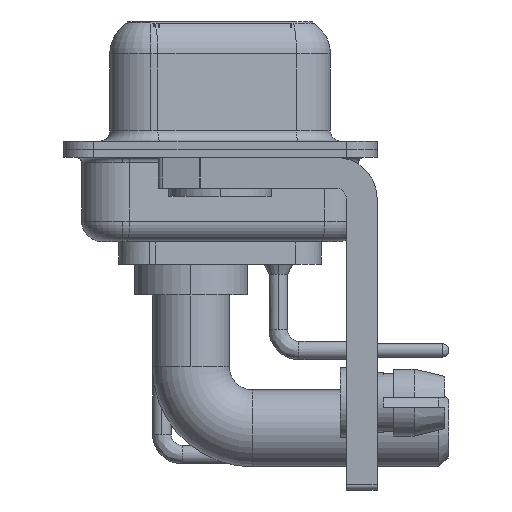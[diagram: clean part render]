
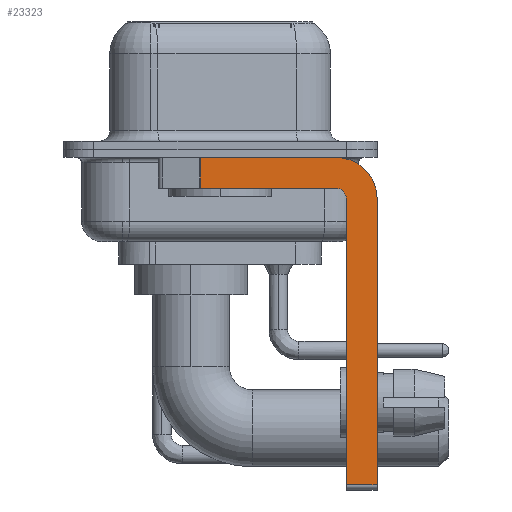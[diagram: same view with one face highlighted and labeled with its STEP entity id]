
A CAD part, left-side view. The second image highlights one B-rep face of the part: STEP entity #23323.
In plain terms, the highlighted planar face has unit normal (-1, 0, 0).
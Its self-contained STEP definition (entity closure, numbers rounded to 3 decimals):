
#7 = LINE ( 'NONE', #16936, #26356 ) ;
#57 = LINE ( 'NONE', #28210, #3231 ) ;
#2900 = LINE ( 'NONE', #16888, #9884 ) ;
#2935 = EDGE_CURVE ( 'NONE', #34196, #8139, #23715, .T. ) ;
#3175 = DIRECTION ( 'NONE',  ( 0., 0., -1. ) ) ;
#3231 = VECTOR ( 'NONE', #3175, 1000. ) ;
#3431 = LINE ( 'NONE', #31217, #35731 ) ;
#4586 = VERTEX_POINT ( 'NONE', #32590 ) ;
#6337 = DIRECTION ( 'NONE',  ( 1., 0., 0. ) ) ;
#8139 = VERTEX_POINT ( 'NONE', #9916 ) ;
#8409 = EDGE_CURVE ( 'NONE', #8139, #26697, #35585, .T. ) ;
#8509 = ORIENTED_EDGE ( 'NONE', *, *, #2935, .F. ) ;
#8805 = ORIENTED_EDGE ( 'NONE', *, *, #31006, .T. ) ;
#9224 = ORIENTED_EDGE ( 'NONE', *, *, #30362, .F. ) ;
#9511 = LINE ( 'NONE', #31940, #32797 ) ;
#9884 = VECTOR ( 'NONE', #13933, 1000. ) ;
#9916 = CARTESIAN_POINT ( 'NONE',  ( -2.9, -5.65, -1.9 ) ) ;
#11908 = EDGE_LOOP ( 'NONE', ( #35743, #8805, #30352, #8509, #9224, #20999, #24292, #25877 ) ) ;
#12571 = DIRECTION ( 'NONE',  ( 0., 0., 1. ) ) ;
#12750 = CARTESIAN_POINT ( 'NONE',  ( -2.9, -5.65, -2.4 ) ) ;
#13039 = CARTESIAN_POINT ( 'NONE',  ( -2.9, -6.15, -2.4 ) ) ;
#13574 = CARTESIAN_POINT ( 'NONE',  ( -2.9, 0.978, -0.4 ) ) ;
#13933 = DIRECTION ( 'NONE',  ( 0., -1., 0. ) ) ;
#14317 = VERTEX_POINT ( 'NONE', #29130 ) ;
#14718 = DIRECTION ( 'NONE',  ( 1., 0., 0. ) ) ;
#15345 = DIRECTION ( 'NONE',  ( -1., 0., 0. ) ) ;
#16706 = DIRECTION ( 'NONE',  ( 0., 0., -1. ) ) ;
#16888 = CARTESIAN_POINT ( 'NONE',  ( -2.9, 3., -0.4 ) ) ;
#16936 = CARTESIAN_POINT ( 'NONE',  ( -2.9, -5.65, -16.35 ) ) ;
#17469 = DIRECTION ( 'NONE',  ( 0., -1., 0. ) ) ;
#18126 = PLANE ( 'NONE',  #21367 ) ;
#18497 = CARTESIAN_POINT ( 'NONE',  ( -2.9, -5.65, -1.9 ) ) ;
#20999 = ORIENTED_EDGE ( 'NONE', *, *, #29851, .T. ) ;
#21367 = AXIS2_PLACEMENT_3D ( 'NONE', #34472, #6337, #31909 ) ;
#21438 = DIRECTION ( 'NONE',  ( 0., 1., 0. ) ) ;
#23323 = ADVANCED_FACE ( 'NONE', ( #31720 ), #18126, .F. ) ;
#23715 = CIRCLE ( 'NONE', #26673, 0.5 ) ;
#24292 = ORIENTED_EDGE ( 'NONE', *, *, #28803, .F. ) ;
#25566 = EDGE_CURVE ( 'NONE', #4586, #31012, #35509, .T. ) ;
#25877 = ORIENTED_EDGE ( 'NONE', *, *, #25566, .F. ) ;
#26356 = VECTOR ( 'NONE', #17469, 1000. ) ;
#26673 = AXIS2_PLACEMENT_3D ( 'NONE', #12750, #15345, #12571 ) ;
#26697 = VERTEX_POINT ( 'NONE', #32928 ) ;
#28210 = CARTESIAN_POINT ( 'NONE',  ( -2.9, 0.978, -1.9 ) ) ;
#28700 = DIRECTION ( 'NONE',  ( 0., 0., -1. ) ) ;
#28803 = EDGE_CURVE ( 'NONE', #31012, #29427, #3431, .T. ) ;
#28882 = CARTESIAN_POINT ( 'NONE',  ( -2.9, -5.65, -2.4 ) ) ;
#29130 = CARTESIAN_POINT ( 'NONE',  ( -2.9, -6.15, -16.35 ) ) ;
#29427 = VERTEX_POINT ( 'NONE', #31841 ) ;
#29851 = EDGE_CURVE ( 'NONE', #14317, #29427, #7, .T. ) ;
#30143 = EDGE_CURVE ( 'NONE', #32949, #4586, #2900, .T. ) ;
#30352 = ORIENTED_EDGE ( 'NONE', *, *, #8409, .F. ) ;
#30362 = EDGE_CURVE ( 'NONE', #14317, #34196, #9511, .T. ) ;
#31006 = EDGE_CURVE ( 'NONE', #32949, #26697, #57, .T. ) ;
#31012 = VERTEX_POINT ( 'NONE', #33511 ) ;
#31040 = VECTOR ( 'NONE', #21438, 1000. ) ;
#31217 = CARTESIAN_POINT ( 'NONE',  ( -2.9, -7.65, -2.4 ) ) ;
#31573 = DIRECTION ( 'NONE',  ( 0., 0., 1. ) ) ;
#31720 = FACE_OUTER_BOUND ( 'NONE', #11908, .T. ) ;
#31841 = CARTESIAN_POINT ( 'NONE',  ( -2.9, -7.65, -16.35 ) ) ;
#31909 = DIRECTION ( 'NONE',  ( 0., 0., -1. ) ) ;
#31940 = CARTESIAN_POINT ( 'NONE',  ( -2.9, -6.15, -16.6 ) ) ;
#32590 = CARTESIAN_POINT ( 'NONE',  ( -2.9, -5.65, -0.4 ) ) ;
#32797 = VECTOR ( 'NONE', #31573, 1000. ) ;
#32928 = CARTESIAN_POINT ( 'NONE',  ( -2.9, 0.978, -1.9 ) ) ;
#32949 = VERTEX_POINT ( 'NONE', #13574 ) ;
#33511 = CARTESIAN_POINT ( 'NONE',  ( -2.9, -7.65, -2.4 ) ) ;
#34196 = VERTEX_POINT ( 'NONE', #13039 ) ;
#34472 = CARTESIAN_POINT ( 'NONE',  ( -2.9, -5.65, -2.4 ) ) ;
#35509 = CIRCLE ( 'NONE', #36109, 2. ) ;
#35585 = LINE ( 'NONE', #18497, #31040 ) ;
#35731 = VECTOR ( 'NONE', #16706, 1000. ) ;
#35743 = ORIENTED_EDGE ( 'NONE', *, *, #30143, .F. ) ;
#36109 = AXIS2_PLACEMENT_3D ( 'NONE', #28882, #14718, #28700 ) ;
